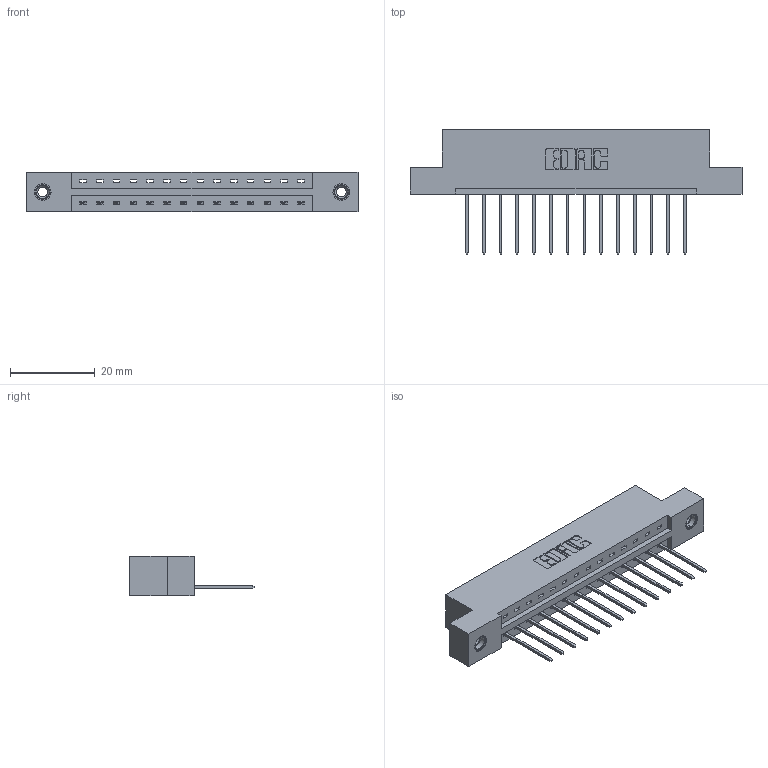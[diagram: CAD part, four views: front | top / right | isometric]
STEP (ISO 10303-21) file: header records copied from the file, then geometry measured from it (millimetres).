
FILE_DESCRIPTION (( 'STEP AP203' ), '1' );
FILE_NAME ('387-014-540-108.STEP', '2018-09-11T04:11:12', ( '' ), ( '' ), 'SwSTEP 2.0', 'SolidWorks 2016', '' );
FILE_SCHEMA (( 'CONFIG_CONTROL_DESIGN' ));
Length unit declared in the file: inch
Products named in the file (4): 337 Part_Flush Mounting Lugs - 0.156 Dia-TI; 345-292-001_345-293-140; 345-250-001_345-250-003-102; 387-014-540-108
Assembly tree (17 placements, depth 2):
  387-014-540-108
    337 Part_Flush Mounting Lugs - 0.156 Dia-TI
    345-292-001_345-293-140  x14
    345-250-001_345-250-003-102  x2
Bounding box: 78.49 x 29.47 x 9.4 mm (x, y, z)
Volume: 7819.4 mm3; surface area: 8095.2 mm2
Topology: 17 solids, 17 shells, 1042 faces, 3079 edges, 2026 vertices
Faces by surface type: plane 746, cylinder 280, cone 12, torus 4
Entity records: 15232 total; most frequent: CARTESIAN_POINT 2631, ORIENTED_EDGE 2574, DIRECTION 2305, EDGE_CURVE 1287, LINE 1139, VECTOR 1139, VERTEX_POINT 852, AXIS2_PLACEMENT_3D 583
